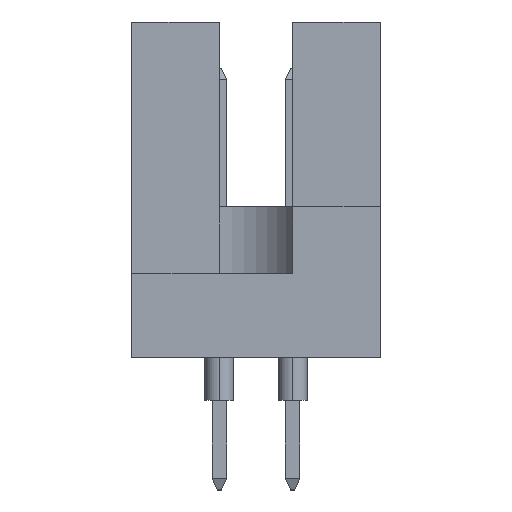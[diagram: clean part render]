
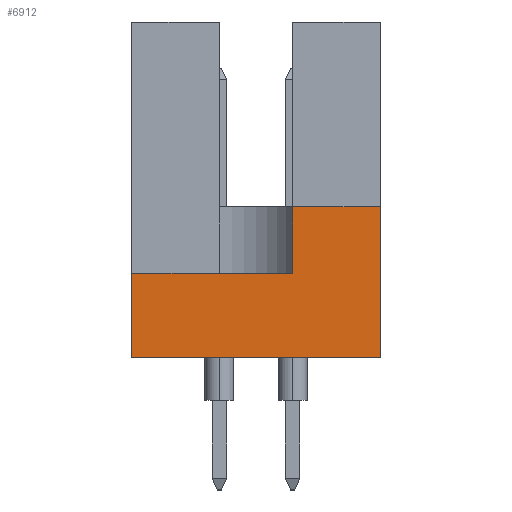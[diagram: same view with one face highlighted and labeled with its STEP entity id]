
A CAD part, left-side view. The second image highlights one B-rep face of the part: STEP entity #6912.
In plain terms, the highlighted planar face has unit normal (-1, 0, 0).
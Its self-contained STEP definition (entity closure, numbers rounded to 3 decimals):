
#340 = VERTEX_POINT ( 'NONE', #5242 ) ;
#390 = ORIENTED_EDGE ( 'NONE', *, *, #11315, .T. ) ;
#622 = VERTEX_POINT ( 'NONE', #12845 ) ;
#719 = VECTOR ( 'NONE', #2204, 1000. ) ;
#971 = AXIS2_PLACEMENT_3D ( 'NONE', #4814, #3683, #6736 ) ;
#2204 = DIRECTION ( 'NONE',  ( 0., 1., 0. ) ) ;
#2225 = CARTESIAN_POINT ( 'NONE',  ( -47.5, -1.27, 5.2 ) ) ;
#2375 = CARTESIAN_POINT ( 'NONE',  ( -47.5, 4.3, 5.2 ) ) ;
#2456 = EDGE_CURVE ( 'NONE', #4169, #4920, #6882, .T. ) ;
#2615 = ORIENTED_EDGE ( 'NONE', *, *, #3865, .T. ) ;
#3546 = CARTESIAN_POINT ( 'NONE',  ( -47.5, -1.27, 2.9 ) ) ;
#3631 = ORIENTED_EDGE ( 'NONE', *, *, #4897, .T. ) ;
#3683 = DIRECTION ( 'NONE',  ( 1., 0., 0. ) ) ;
#3716 = VECTOR ( 'NONE', #7423, 1000. ) ;
#3786 = EDGE_CURVE ( 'NONE', #4412, #7143, #4724, .T. ) ;
#3861 = CARTESIAN_POINT ( 'NONE',  ( -47.5, 4.3, 11.6 ) ) ;
#3865 = EDGE_CURVE ( 'NONE', #622, #340, #4863, .T. ) ;
#3902 = ORIENTED_EDGE ( 'NONE', *, *, #6115, .F. ) ;
#4071 = LINE ( 'NONE', #9255, #719 ) ;
#4169 = VERTEX_POINT ( 'NONE', #6616 ) ;
#4209 = CARTESIAN_POINT ( 'NONE',  ( -47.5, 4.3, 0. ) ) ;
#4412 = VERTEX_POINT ( 'NONE', #2225 ) ;
#4724 = LINE ( 'NONE', #11954, #4822 ) ;
#4814 = CARTESIAN_POINT ( 'NONE',  ( -47.5, 4.3, 11.6 ) ) ;
#4822 = VECTOR ( 'NONE', #5782, 1000. ) ;
#4863 = LINE ( 'NONE', #3861, #8558 ) ;
#4897 = EDGE_CURVE ( 'NONE', #7143, #622, #4071, .T. ) ;
#4920 = VERTEX_POINT ( 'NONE', #5344 ) ;
#4945 = ORIENTED_EDGE ( 'NONE', *, *, #3786, .T. ) ;
#5242 = CARTESIAN_POINT ( 'NONE',  ( -47.5, 4.3, 0. ) ) ;
#5344 = CARTESIAN_POINT ( 'NONE',  ( -47.5, -4.3, 0. ) ) ;
#5782 = DIRECTION ( 'NONE',  ( 0., 0., -1. ) ) ;
#6115 = EDGE_CURVE ( 'NONE', #4412, #4169, #10543, .T. ) ;
#6452 = VECTOR ( 'NONE', #6818, 1000. ) ;
#6616 = CARTESIAN_POINT ( 'NONE',  ( -47.5, -4.3, 5.2 ) ) ;
#6736 = DIRECTION ( 'NONE',  ( 0., 0., -1. ) ) ;
#6818 = DIRECTION ( 'NONE',  ( 0., 0., -1. ) ) ;
#6882 = LINE ( 'NONE', #11075, #6452 ) ;
#6912 = ADVANCED_FACE ( 'NONE', ( #7725 ), #12776, .F. ) ;
#7143 = VERTEX_POINT ( 'NONE', #3546 ) ;
#7423 = DIRECTION ( 'NONE',  ( 0., -1., 0. ) ) ;
#7725 = FACE_OUTER_BOUND ( 'NONE', #12374, .T. ) ;
#8430 = VECTOR ( 'NONE', #10570, 1000. ) ;
#8558 = VECTOR ( 'NONE', #8910, 1000. ) ;
#8910 = DIRECTION ( 'NONE',  ( 0., 0., -1. ) ) ;
#9255 = CARTESIAN_POINT ( 'NONE',  ( -47.5, 4.3, 2.9 ) ) ;
#10382 = LINE ( 'NONE', #4209, #8430 ) ;
#10404 = ORIENTED_EDGE ( 'NONE', *, *, #2456, .F. ) ;
#10543 = LINE ( 'NONE', #2375, #3716 ) ;
#10570 = DIRECTION ( 'NONE',  ( 0., -1., 0. ) ) ;
#11075 = CARTESIAN_POINT ( 'NONE',  ( -47.5, -4.3, 11.6 ) ) ;
#11315 = EDGE_CURVE ( 'NONE', #340, #4920, #10382, .T. ) ;
#11954 = CARTESIAN_POINT ( 'NONE',  ( -47.5, -1.27, 19.02 ) ) ;
#12374 = EDGE_LOOP ( 'NONE', ( #3902, #4945, #3631, #2615, #390, #10404 ) ) ;
#12776 = PLANE ( 'NONE',  #971 ) ;
#12845 = CARTESIAN_POINT ( 'NONE',  ( -47.5, 4.3, 2.9 ) ) ;
